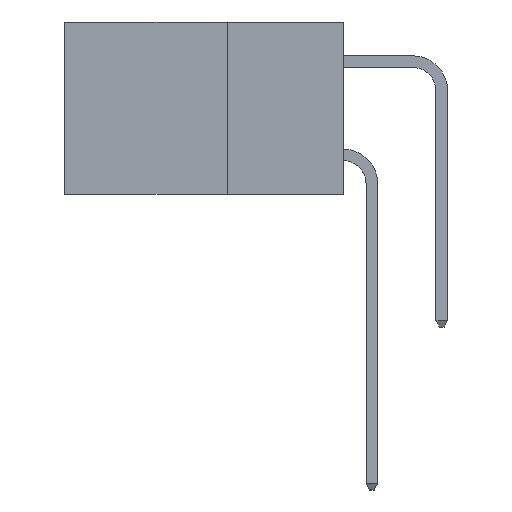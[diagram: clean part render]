
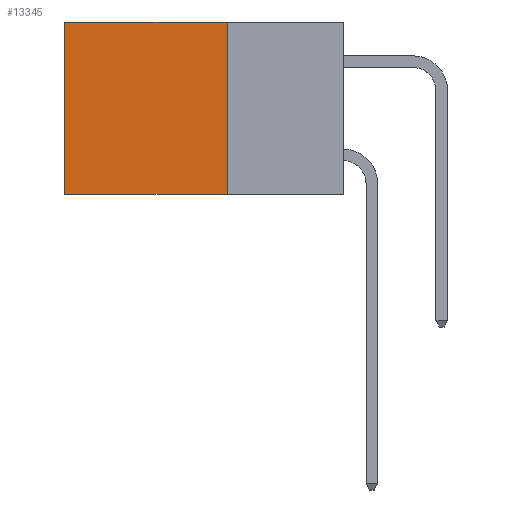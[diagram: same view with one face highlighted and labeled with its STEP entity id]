
A CAD part, left-side view. The second image highlights one B-rep face of the part: STEP entity #13345.
In plain terms, the highlighted planar face has unit normal (-1, 0, 0).
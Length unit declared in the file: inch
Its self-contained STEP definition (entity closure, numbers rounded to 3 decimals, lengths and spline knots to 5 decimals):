
#1350 = CARTESIAN_POINT ( 'NONE',  ( 0.2615, 0.25, -0.37 ) ) ;
#1611 = VECTOR ( 'NONE', #13652, 39.37008 ) ;
#1669 = DIRECTION ( 'NONE',  ( 0., 0., -1. ) ) ;
#2020 = AXIS2_PLACEMENT_3D ( 'NONE', #2514, #10001, #3582 ) ;
#2278 = LINE ( 'NONE', #3952, #7657 ) ;
#2514 = CARTESIAN_POINT ( 'NONE',  ( 0.2615, 0.25, -0.37 ) ) ;
#2605 = CARTESIAN_POINT ( 'NONE',  ( 0.2615, 0.25, -0.37 ) ) ;
#2850 = FACE_OUTER_BOUND ( 'NONE', #3098, .T. ) ;
#3098 = EDGE_LOOP ( 'NONE', ( #12020, #6793, #4107, #8659 ) ) ;
#3582 = DIRECTION ( 'NONE',  ( 0., 0., -1. ) ) ;
#3695 = DIRECTION ( 'NONE',  ( 0., 0., -1. ) ) ;
#3952 = CARTESIAN_POINT ( 'NONE',  ( 0.2615, 0.6, -0.37 ) ) ;
#4107 = ORIENTED_EDGE ( 'NONE', *, *, #5553, .F. ) ;
#4241 = CARTESIAN_POINT ( 'NONE',  ( 0.2615, 0.6, 0. ) ) ;
#4518 = LINE ( 'NONE', #13496, #1611 ) ;
#4722 = EDGE_CURVE ( 'NONE', #12029, #13450, #2278, .T. ) ;
#4772 = VERTEX_POINT ( 'NONE', #2605 ) ;
#5553 = EDGE_CURVE ( 'NONE', #11867, #4772, #11155, .T. ) ;
#5779 = CARTESIAN_POINT ( 'NONE',  ( 0.2615, 0.25, 0. ) ) ;
#5935 = CARTESIAN_POINT ( 'NONE',  ( 0.2615, 0.25, 0. ) ) ;
#6131 = DIRECTION ( 'NONE',  ( 0., 1., 0. ) ) ;
#6793 = ORIENTED_EDGE ( 'NONE', *, *, #9733, .F. ) ;
#7617 = VECTOR ( 'NONE', #6131, 39.37008 ) ;
#7657 = VECTOR ( 'NONE', #3695, 39.37008 ) ;
#8605 = EDGE_CURVE ( 'NONE', #11867, #12029, #10452, .T. ) ;
#8659 = ORIENTED_EDGE ( 'NONE', *, *, #8605, .T. ) ;
#8924 = PLANE ( 'NONE',  #2020 ) ;
#9733 = EDGE_CURVE ( 'NONE', #4772, #13450, #4518, .T. ) ;
#10001 = DIRECTION ( 'NONE',  ( 1., 0., 0. ) ) ;
#10452 = LINE ( 'NONE', #5935, #7617 ) ;
#10801 = VECTOR ( 'NONE', #1669, 39.37008 ) ;
#11155 = LINE ( 'NONE', #1350, #10801 ) ;
#11867 = VERTEX_POINT ( 'NONE', #5779 ) ;
#12020 = ORIENTED_EDGE ( 'NONE', *, *, #4722, .T. ) ;
#12029 = VERTEX_POINT ( 'NONE', #4241 ) ;
#13345 = ADVANCED_FACE ( 'NONE', ( #2850 ), #8924, .F. ) ;
#13352 = CARTESIAN_POINT ( 'NONE',  ( 0.2615, 0.6, -0.37 ) ) ;
#13450 = VERTEX_POINT ( 'NONE', #13352 ) ;
#13496 = CARTESIAN_POINT ( 'NONE',  ( 0.2615, 0.25, -0.37 ) ) ;
#13652 = DIRECTION ( 'NONE',  ( 0., 1., 0. ) ) ;
